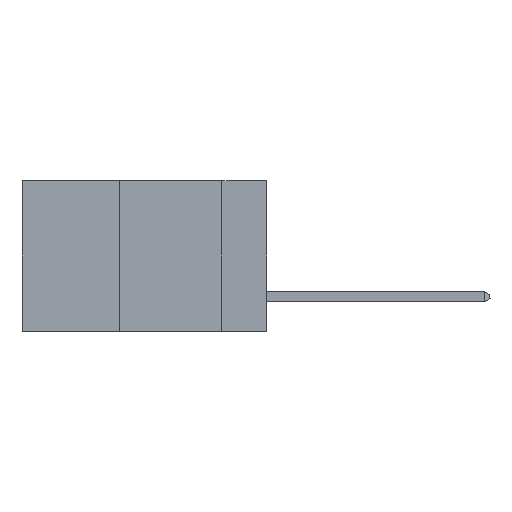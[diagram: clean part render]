
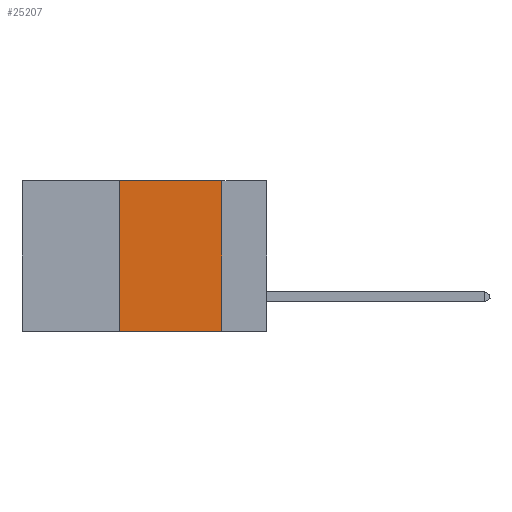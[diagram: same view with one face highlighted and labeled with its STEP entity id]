
A CAD part, left-side view. The second image highlights one B-rep face of the part: STEP entity #25207.
In plain terms, the highlighted planar face has unit normal (-1, 0, 0).
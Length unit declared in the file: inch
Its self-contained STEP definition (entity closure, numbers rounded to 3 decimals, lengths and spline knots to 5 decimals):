
#205 = DIRECTION ( 'NONE',  ( 1., 0., 0. ) ) ;
#1033 = CARTESIAN_POINT ( 'NONE',  ( 0., 0.36, 0. ) ) ;
#2133 = VERTEX_POINT ( 'NONE', #19012 ) ;
#2737 = CARTESIAN_POINT ( 'NONE',  ( 0., 0.6, 0. ) ) ;
#2843 = VECTOR ( 'NONE', #30894, 39.37008 ) ;
#3244 = VERTEX_POINT ( 'NONE', #27033 ) ;
#5363 = CARTESIAN_POINT ( 'NONE',  ( 0., 0.11, 0. ) ) ;
#5591 = FACE_OUTER_BOUND ( 'NONE', #20453, .T. ) ;
#5635 = EDGE_CURVE ( 'NONE', #2133, #3244, #19142, .T. ) ;
#5998 = EDGE_CURVE ( 'NONE', #26746, #28415, #34909, .T. ) ;
#9706 = CARTESIAN_POINT ( 'NONE',  ( 0., 0.11, 0. ) ) ;
#10089 = AXIS2_PLACEMENT_3D ( 'NONE', #2737, #205, #19381 ) ;
#11765 = CARTESIAN_POINT ( 'NONE',  ( 0., 0.6, -0.37 ) ) ;
#12856 = DIRECTION ( 'NONE',  ( 0., 0., 1. ) ) ;
#13600 = ORIENTED_EDGE ( 'NONE', *, *, #5998, .F. ) ;
#15704 = VECTOR ( 'NONE', #23711, 39.37008 ) ;
#16437 = DIRECTION ( 'NONE',  ( 0., -1., 0. ) ) ;
#19012 = CARTESIAN_POINT ( 'NONE',  ( 0., 0.36, -0.37 ) ) ;
#19127 = LINE ( 'NONE', #9706, #15704 ) ;
#19142 = LINE ( 'NONE', #11765, #2843 ) ;
#19381 = DIRECTION ( 'NONE',  ( 0., 0., -1. ) ) ;
#20453 = EDGE_LOOP ( 'NONE', ( #31769, #13600, #24403, #25612 ) ) ;
#23711 = DIRECTION ( 'NONE',  ( 0., 0., -1. ) ) ;
#24403 = ORIENTED_EDGE ( 'NONE', *, *, #25559, .F. ) ;
#24769 = CARTESIAN_POINT ( 'NONE',  ( 0., 0.6, 0. ) ) ;
#25207 = ADVANCED_FACE ( 'NONE', ( #5591 ), #32975, .F. ) ;
#25559 = EDGE_CURVE ( 'NONE', #2133, #26746, #26097, .T. ) ;
#25612 = ORIENTED_EDGE ( 'NONE', *, *, #5635, .T. ) ;
#26097 = LINE ( 'NONE', #26357, #29077 ) ;
#26357 = CARTESIAN_POINT ( 'NONE',  ( 0., 0.36, 0. ) ) ;
#26746 = VERTEX_POINT ( 'NONE', #1033 ) ;
#27033 = CARTESIAN_POINT ( 'NONE',  ( 0., 0.11, -0.37 ) ) ;
#28415 = VERTEX_POINT ( 'NONE', #5363 ) ;
#29077 = VECTOR ( 'NONE', #12856, 39.37008 ) ;
#30894 = DIRECTION ( 'NONE',  ( 0., -1., 0. ) ) ;
#31769 = ORIENTED_EDGE ( 'NONE', *, *, #33657, .F. ) ;
#32975 = PLANE ( 'NONE',  #10089 ) ;
#33657 = EDGE_CURVE ( 'NONE', #28415, #3244, #19127, .T. ) ;
#34057 = VECTOR ( 'NONE', #16437, 39.37008 ) ;
#34909 = LINE ( 'NONE', #24769, #34057 ) ;
